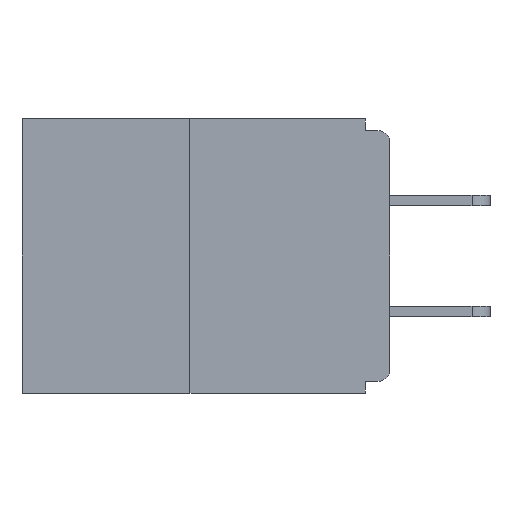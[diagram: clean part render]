
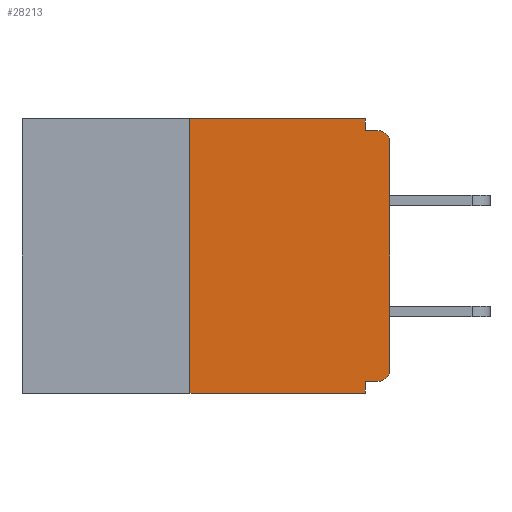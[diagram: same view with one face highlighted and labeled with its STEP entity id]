
A CAD part, left-side view. The second image highlights one B-rep face of the part: STEP entity #28213.
In plain terms, the highlighted planar face has unit normal (-1, 0, 0).
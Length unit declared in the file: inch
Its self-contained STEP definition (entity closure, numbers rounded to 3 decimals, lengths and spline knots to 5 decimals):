
#936 = EDGE_CURVE ( 'NONE', #13210, #17508, #5033, .T. ) ;
#1382 = EDGE_CURVE ( 'NONE', #22806, #9765, #3606, .T. ) ;
#1453 = DIRECTION ( 'NONE',  ( 0., 0., -1. ) ) ;
#1815 = VERTEX_POINT ( 'NONE', #20308 ) ;
#1970 = EDGE_CURVE ( 'NONE', #17508, #8468, #8156, .T. ) ;
#2792 = VERTEX_POINT ( 'NONE', #4309 ) ;
#2913 = DIRECTION ( 'NONE',  ( 0., 0., -1. ) ) ;
#2979 = LINE ( 'NONE', #14961, #9626 ) ;
#3164 = DIRECTION ( 'NONE',  ( 0., -1., 0. ) ) ;
#3387 = CARTESIAN_POINT ( 'NONE',  ( 0., 0., -0.313 ) ) ;
#3606 = LINE ( 'NONE', #20292, #18335 ) ;
#4309 = CARTESIAN_POINT ( 'NONE',  ( 0., 0.25, -0.343 ) ) ;
#4797 = ORIENTED_EDGE ( 'NONE', *, *, #1970, .T. ) ;
#5033 = CIRCLE ( 'NONE', #15910, 0.015 ) ;
#6063 = PLANE ( 'NONE',  #6144 ) ;
#6144 = AXIS2_PLACEMENT_3D ( 'NONE', #21752, #21658, #22330 ) ;
#7626 = VERTEX_POINT ( 'NONE', #8536 ) ;
#7804 = ORIENTED_EDGE ( 'NONE', *, *, #18376, .F. ) ;
#8140 = DIRECTION ( 'NONE',  ( 0., 0., 1. ) ) ;
#8155 = VERTEX_POINT ( 'NONE', #9800 ) ;
#8156 = LINE ( 'NONE', #16882, #20767 ) ;
#8170 = ORIENTED_EDGE ( 'NONE', *, *, #14051, .F. ) ;
#8190 = DIRECTION ( 'NONE',  ( 0., 0., -1. ) ) ;
#8285 = DIRECTION ( 'NONE',  ( -1., 0., 0. ) ) ;
#8468 = VERTEX_POINT ( 'NONE', #13681 ) ;
#8536 = CARTESIAN_POINT ( 'NONE',  ( 0., 0.015, -0.015 ) ) ;
#8913 = EDGE_CURVE ( 'NONE', #15334, #1815, #15725, .T. ) ;
#9067 = VECTOR ( 'NONE', #2913, 39.37008 ) ;
#9580 = CARTESIAN_POINT ( 'NONE',  ( 0., 0.015, -0.03 ) ) ;
#9626 = VECTOR ( 'NONE', #23792, 39.37008 ) ;
#9765 = VERTEX_POINT ( 'NONE', #19471 ) ;
#9800 = CARTESIAN_POINT ( 'NONE',  ( 0., 0.25, 0. ) ) ;
#9915 = EDGE_CURVE ( 'NONE', #13210, #22806, #23391, .T. ) ;
#9946 = VECTOR ( 'NONE', #3164, 39.37008 ) ;
#11144 = VECTOR ( 'NONE', #20033, 39.37008 ) ;
#11610 = ORIENTED_EDGE ( 'NONE', *, *, #9915, .F. ) ;
#11653 = DIRECTION ( 'NONE',  ( 0., 0., -1. ) ) ;
#11743 = ORIENTED_EDGE ( 'NONE', *, *, #20135, .T. ) ;
#11965 = ORIENTED_EDGE ( 'NONE', *, *, #1382, .F. ) ;
#12193 = AXIS2_PLACEMENT_3D ( 'NONE', #9580, #23022, #11653 ) ;
#13210 = VERTEX_POINT ( 'NONE', #14491 ) ;
#13220 = VECTOR ( 'NONE', #14168, 39.37008 ) ;
#13681 = CARTESIAN_POINT ( 'NONE',  ( 0., 0., -0.03 ) ) ;
#13890 = VECTOR ( 'NONE', #8140, 39.37008 ) ;
#14051 = EDGE_CURVE ( 'NONE', #8155, #15334, #25726, .T. ) ;
#14168 = DIRECTION ( 'NONE',  ( 0., 1., 0. ) ) ;
#14491 = CARTESIAN_POINT ( 'NONE',  ( 0., 0.015, -0.328 ) ) ;
#14866 = ORIENTED_EDGE ( 'NONE', *, *, #936, .T. ) ;
#14961 = CARTESIAN_POINT ( 'NONE',  ( 0., 0., -0.015 ) ) ;
#15334 = VERTEX_POINT ( 'NONE', #16165 ) ;
#15725 = LINE ( 'NONE', #18807, #9067 ) ;
#15910 = AXIS2_PLACEMENT_3D ( 'NONE', #23890, #8285, #1453 ) ;
#16165 = CARTESIAN_POINT ( 'NONE',  ( 0., 0.031, 0. ) ) ;
#16369 = LINE ( 'NONE', #21574, #13890 ) ;
#16882 = CARTESIAN_POINT ( 'NONE',  ( 0., 0., 0. ) ) ;
#17116 = LINE ( 'NONE', #28535, #11144 ) ;
#17508 = VERTEX_POINT ( 'NONE', #3387 ) ;
#17752 = EDGE_CURVE ( 'NONE', #2792, #9765, #17116, .T. ) ;
#18315 = CARTESIAN_POINT ( 'NONE',  ( 0., 0.031, -0.328 ) ) ;
#18335 = VECTOR ( 'NONE', #8190, 39.37008 ) ;
#18376 = EDGE_CURVE ( 'NONE', #2792, #8155, #16369, .T. ) ;
#18807 = CARTESIAN_POINT ( 'NONE',  ( 0., 0.031, 0. ) ) ;
#19471 = CARTESIAN_POINT ( 'NONE',  ( 0., 0.031, -0.343 ) ) ;
#19651 = EDGE_CURVE ( 'NONE', #1815, #7626, #2979, .T. ) ;
#19673 = ORIENTED_EDGE ( 'NONE', *, *, #17752, .T. ) ;
#20033 = DIRECTION ( 'NONE',  ( 0., -1., 0. ) ) ;
#20135 = EDGE_CURVE ( 'NONE', #8468, #7626, #26775, .T. ) ;
#20292 = CARTESIAN_POINT ( 'NONE',  ( 0., 0.031, -0.343 ) ) ;
#20308 = CARTESIAN_POINT ( 'NONE',  ( 0., 0.031, -0.015 ) ) ;
#20670 = ORIENTED_EDGE ( 'NONE', *, *, #19651, .F. ) ;
#20767 = VECTOR ( 'NONE', #21684, 39.37008 ) ;
#21574 = CARTESIAN_POINT ( 'NONE',  ( 0., 0.25, 0. ) ) ;
#21658 = DIRECTION ( 'NONE',  ( 1., 0., 0. ) ) ;
#21684 = DIRECTION ( 'NONE',  ( 0., 0., 1. ) ) ;
#21752 = CARTESIAN_POINT ( 'NONE',  ( 0., 0.46, 0. ) ) ;
#22330 = DIRECTION ( 'NONE',  ( 0., 0., -1. ) ) ;
#22806 = VERTEX_POINT ( 'NONE', #18315 ) ;
#23022 = DIRECTION ( 'NONE',  ( -1., 0., 0. ) ) ;
#23149 = EDGE_LOOP ( 'NONE', ( #8170, #7804, #19673, #11965, #11610, #14866, #4797, #11743, #20670, #27673 ) ) ;
#23391 = LINE ( 'NONE', #27572, #13220 ) ;
#23557 = CARTESIAN_POINT ( 'NONE',  ( 0., 0.46, 0. ) ) ;
#23792 = DIRECTION ( 'NONE',  ( 0., -1., 0. ) ) ;
#23890 = CARTESIAN_POINT ( 'NONE',  ( 0., 0.015, -0.313 ) ) ;
#25620 = FACE_OUTER_BOUND ( 'NONE', #23149, .T. ) ;
#25726 = LINE ( 'NONE', #23557, #9946 ) ;
#26775 = CIRCLE ( 'NONE', #12193, 0.015 ) ;
#27572 = CARTESIAN_POINT ( 'NONE',  ( 0., 0., -0.328 ) ) ;
#27673 = ORIENTED_EDGE ( 'NONE', *, *, #8913, .F. ) ;
#28213 = ADVANCED_FACE ( 'NONE', ( #25620 ), #6063, .F. ) ;
#28535 = CARTESIAN_POINT ( 'NONE',  ( 0., 0.46, -0.343 ) ) ;
